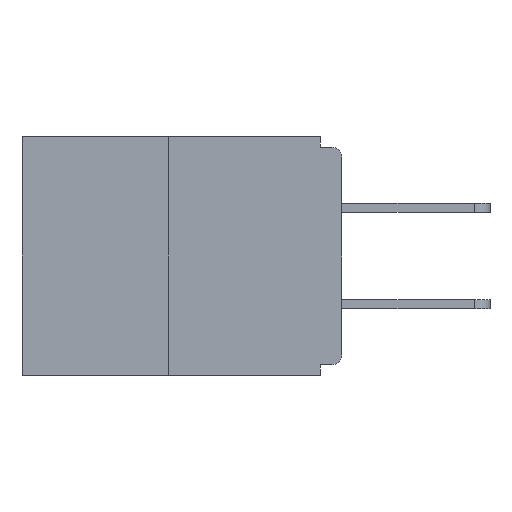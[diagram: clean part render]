
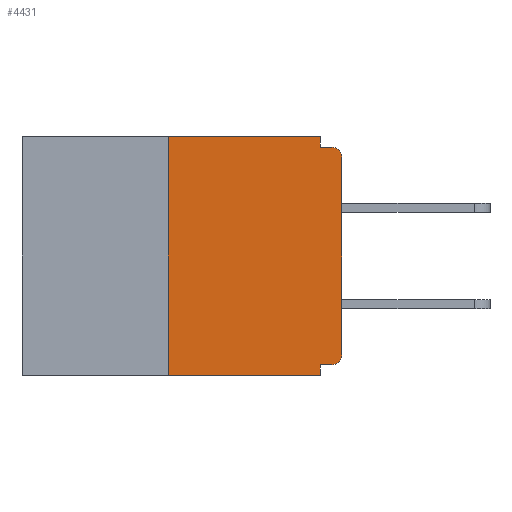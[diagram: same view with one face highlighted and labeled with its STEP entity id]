
A CAD part, left-side view. The second image highlights one B-rep face of the part: STEP entity #4431.
In plain terms, the highlighted planar face has unit normal (-1, 0, 0).
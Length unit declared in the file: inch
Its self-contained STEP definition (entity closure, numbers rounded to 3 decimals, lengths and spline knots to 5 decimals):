
#1232 = LINE ( 'NONE', #15457, #12209 ) ;
#1467 = EDGE_CURVE ( 'NONE', #7406, #3227, #15277, .T. ) ;
#1513 = CARTESIAN_POINT ( 'NONE',  ( 0., 0., -0.015 ) ) ;
#1574 = DIRECTION ( 'NONE',  ( 0., 0., -1. ) ) ;
#1651 = VERTEX_POINT ( 'NONE', #2709 ) ;
#2581 = CARTESIAN_POINT ( 'NONE',  ( 0., 0., -0.328 ) ) ;
#2709 = CARTESIAN_POINT ( 'NONE',  ( 0., 0.031, 0. ) ) ;
#2774 = ORIENTED_EDGE ( 'NONE', *, *, #5247, .T. ) ;
#2903 = PLANE ( 'NONE',  #15243 ) ;
#3227 = VERTEX_POINT ( 'NONE', #6611 ) ;
#3639 = CARTESIAN_POINT ( 'NONE',  ( 0., 0.015, -0.03 ) ) ;
#3704 = DIRECTION ( 'NONE',  ( 0., 0., -1. ) ) ;
#3724 = VERTEX_POINT ( 'NONE', #17687 ) ;
#3806 = CARTESIAN_POINT ( 'NONE',  ( 0., 0.031, -0.328 ) ) ;
#4276 = DIRECTION ( 'NONE',  ( 0., -1., 0. ) ) ;
#4431 = ADVANCED_FACE ( 'NONE', ( #5269 ), #2903, .F. ) ;
#4559 = LINE ( 'NONE', #14649, #17746 ) ;
#4622 = CARTESIAN_POINT ( 'NONE',  ( 0., 0.015, -0.328 ) ) ;
#4628 = DIRECTION ( 'NONE',  ( 1., 0., 0. ) ) ;
#4949 = DIRECTION ( 'NONE',  ( 0., -1., 0. ) ) ;
#5142 = DIRECTION ( 'NONE',  ( 0., 0., -1. ) ) ;
#5247 = EDGE_CURVE ( 'NONE', #16214, #8261, #8187, .T. ) ;
#5269 = FACE_OUTER_BOUND ( 'NONE', #6448, .T. ) ;
#5687 = DIRECTION ( 'NONE',  ( 0., 0., -1. ) ) ;
#5733 = CARTESIAN_POINT ( 'NONE',  ( 0., 0.25, 0. ) ) ;
#5944 = EDGE_CURVE ( 'NONE', #16214, #7919, #11638, .T. ) ;
#6207 = LINE ( 'NONE', #20232, #20178 ) ;
#6448 = EDGE_LOOP ( 'NONE', ( #7253, #20790, #7222, #13095, #19895, #2774, #16042, #21369, #15991, #19066 ) ) ;
#6572 = VECTOR ( 'NONE', #14632, 39.37008 ) ;
#6611 = CARTESIAN_POINT ( 'NONE',  ( 0., 0.031, -0.343 ) ) ;
#7222 = ORIENTED_EDGE ( 'NONE', *, *, #1467, .T. ) ;
#7253 = ORIENTED_EDGE ( 'NONE', *, *, #8662, .F. ) ;
#7307 = CARTESIAN_POINT ( 'NONE',  ( 0., 0.015, -0.015 ) ) ;
#7406 = VERTEX_POINT ( 'NONE', #10577 ) ;
#7919 = VERTEX_POINT ( 'NONE', #3806 ) ;
#8187 = CIRCLE ( 'NONE', #19265, 0.015 ) ;
#8261 = VERTEX_POINT ( 'NONE', #22008 ) ;
#8662 = EDGE_CURVE ( 'NONE', #12980, #1651, #4559, .T. ) ;
#8970 = DIRECTION ( 'NONE',  ( -1., 0., 0. ) ) ;
#9736 = EDGE_CURVE ( 'NONE', #21475, #15779, #10192, .T. ) ;
#9836 = VECTOR ( 'NONE', #5142, 39.37008 ) ;
#9967 = LINE ( 'NONE', #5733, #16171 ) ;
#10192 = CIRCLE ( 'NONE', #15306, 0.015 ) ;
#10577 = CARTESIAN_POINT ( 'NONE',  ( 0., 0.25, -0.343 ) ) ;
#10711 = CARTESIAN_POINT ( 'NONE',  ( 0., 0.015, -0.313 ) ) ;
#11638 = LINE ( 'NONE', #2581, #6572 ) ;
#12209 = VECTOR ( 'NONE', #15307, 39.37008 ) ;
#12509 = EDGE_CURVE ( 'NONE', #7406, #12980, #9967, .T. ) ;
#12826 = EDGE_CURVE ( 'NONE', #7919, #3227, #6207, .T. ) ;
#12980 = VERTEX_POINT ( 'NONE', #19497 ) ;
#13095 = ORIENTED_EDGE ( 'NONE', *, *, #12826, .F. ) ;
#14032 = DIRECTION ( 'NONE',  ( -1., 0., 0. ) ) ;
#14632 = DIRECTION ( 'NONE',  ( 0., 1., 0. ) ) ;
#14649 = CARTESIAN_POINT ( 'NONE',  ( 0., 0.46, 0. ) ) ;
#15232 = LINE ( 'NONE', #19972, #9836 ) ;
#15243 = AXIS2_PLACEMENT_3D ( 'NONE', #16441, #4628, #21578 ) ;
#15277 = LINE ( 'NONE', #16180, #22292 ) ;
#15306 = AXIS2_PLACEMENT_3D ( 'NONE', #3639, #14032, #3704 ) ;
#15307 = DIRECTION ( 'NONE',  ( 0., 0., 1. ) ) ;
#15345 = EDGE_CURVE ( 'NONE', #1651, #3724, #15232, .T. ) ;
#15457 = CARTESIAN_POINT ( 'NONE',  ( 0., 0., 0. ) ) ;
#15779 = VERTEX_POINT ( 'NONE', #7307 ) ;
#15991 = ORIENTED_EDGE ( 'NONE', *, *, #16621, .F. ) ;
#16042 = ORIENTED_EDGE ( 'NONE', *, *, #19473, .T. ) ;
#16047 = DIRECTION ( 'NONE',  ( 0., 0., 1. ) ) ;
#16171 = VECTOR ( 'NONE', #16047, 39.37008 ) ;
#16180 = CARTESIAN_POINT ( 'NONE',  ( 0., 0.46, -0.343 ) ) ;
#16214 = VERTEX_POINT ( 'NONE', #4622 ) ;
#16441 = CARTESIAN_POINT ( 'NONE',  ( 0., 0.46, 0. ) ) ;
#16621 = EDGE_CURVE ( 'NONE', #3724, #15779, #21290, .T. ) ;
#16710 = VECTOR ( 'NONE', #4949, 39.37008 ) ;
#17687 = CARTESIAN_POINT ( 'NONE',  ( 0., 0.031, -0.015 ) ) ;
#17746 = VECTOR ( 'NONE', #21802, 39.37008 ) ;
#17807 = CARTESIAN_POINT ( 'NONE',  ( 0., 0., -0.03 ) ) ;
#19066 = ORIENTED_EDGE ( 'NONE', *, *, #15345, .F. ) ;
#19265 = AXIS2_PLACEMENT_3D ( 'NONE', #10711, #8970, #5687 ) ;
#19473 = EDGE_CURVE ( 'NONE', #8261, #21475, #1232, .T. ) ;
#19497 = CARTESIAN_POINT ( 'NONE',  ( 0., 0.25, 0. ) ) ;
#19895 = ORIENTED_EDGE ( 'NONE', *, *, #5944, .F. ) ;
#19972 = CARTESIAN_POINT ( 'NONE',  ( 0., 0.031, 0. ) ) ;
#20178 = VECTOR ( 'NONE', #1574, 39.37008 ) ;
#20232 = CARTESIAN_POINT ( 'NONE',  ( 0., 0.031, -0.343 ) ) ;
#20790 = ORIENTED_EDGE ( 'NONE', *, *, #12509, .F. ) ;
#21290 = LINE ( 'NONE', #1513, #16710 ) ;
#21369 = ORIENTED_EDGE ( 'NONE', *, *, #9736, .T. ) ;
#21475 = VERTEX_POINT ( 'NONE', #17807 ) ;
#21578 = DIRECTION ( 'NONE',  ( 0., 0., -1. ) ) ;
#21802 = DIRECTION ( 'NONE',  ( 0., -1., 0. ) ) ;
#22008 = CARTESIAN_POINT ( 'NONE',  ( 0., 0., -0.313 ) ) ;
#22292 = VECTOR ( 'NONE', #4276, 39.37008 ) ;
